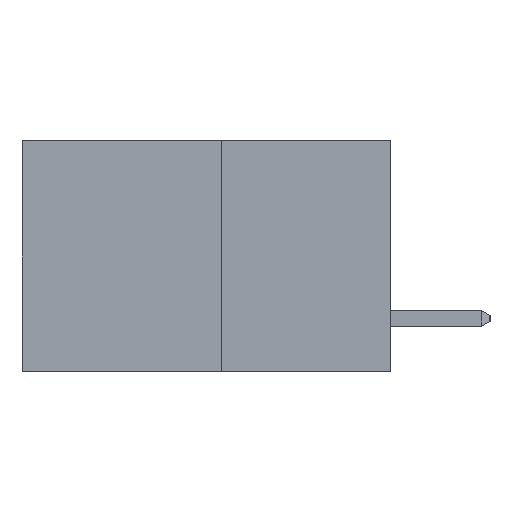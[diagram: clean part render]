
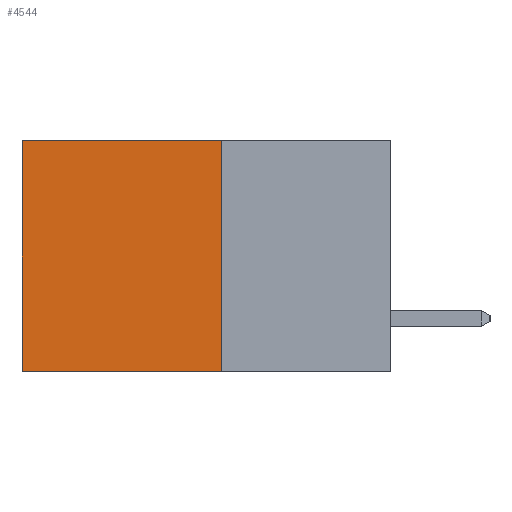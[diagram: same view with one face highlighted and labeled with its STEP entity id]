
A CAD part, left-side view. The second image highlights one B-rep face of the part: STEP entity #4544.
In plain terms, the highlighted planar face has unit normal (-1, 0, 0).
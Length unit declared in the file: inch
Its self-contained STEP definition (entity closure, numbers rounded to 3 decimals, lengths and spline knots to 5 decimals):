
#632 = ORIENTED_EDGE ( 'NONE', *, *, #2432, .T. ) ;
#1020 = VERTEX_POINT ( 'NONE', #12613 ) ;
#1142 = LINE ( 'NONE', #11626, #12280 ) ;
#2432 = EDGE_CURVE ( 'NONE', #9620, #4138, #7521, .T. ) ;
#3687 = VECTOR ( 'NONE', #4342, 39.37008 ) ;
#4007 = ORIENTED_EDGE ( 'NONE', *, *, #14907, .F. ) ;
#4138 = VERTEX_POINT ( 'NONE', #17553 ) ;
#4262 = DIRECTION ( 'NONE',  ( 1., 0., 0. ) ) ;
#4342 = DIRECTION ( 'NONE',  ( 0., 0., -1. ) ) ;
#4544 = ADVANCED_FACE ( 'NONE', ( #16611 ), #11403, .F. ) ;
#4666 = CARTESIAN_POINT ( 'NONE',  ( 0.277, 0.27, 0. ) ) ;
#5407 = EDGE_LOOP ( 'NONE', ( #8310, #11343, #4007, #632 ) ) ;
#7521 = LINE ( 'NONE', #11103, #14602 ) ;
#7532 = LINE ( 'NONE', #10009, #3687 ) ;
#7686 = LINE ( 'NONE', #16466, #8535 ) ;
#7999 = DIRECTION ( 'NONE',  ( 0., 0., -1. ) ) ;
#8310 = ORIENTED_EDGE ( 'NONE', *, *, #10918, .T. ) ;
#8503 = CARTESIAN_POINT ( 'NONE',  ( 0.277, 0.27, -0.37 ) ) ;
#8535 = VECTOR ( 'NONE', #7999, 39.37008 ) ;
#9078 = VERTEX_POINT ( 'NONE', #14856 ) ;
#9620 = VERTEX_POINT ( 'NONE', #4666 ) ;
#10009 = CARTESIAN_POINT ( 'NONE',  ( 0.277, 0.27, -0.37 ) ) ;
#10918 = EDGE_CURVE ( 'NONE', #4138, #9078, #7686, .T. ) ;
#11103 = CARTESIAN_POINT ( 'NONE',  ( 0.277, 0.27, 0. ) ) ;
#11343 = ORIENTED_EDGE ( 'NONE', *, *, #13073, .F. ) ;
#11403 = PLANE ( 'NONE',  #17893 ) ;
#11626 = CARTESIAN_POINT ( 'NONE',  ( 0.277, 0.27, -0.37 ) ) ;
#12280 = VECTOR ( 'NONE', #15766, 39.37008 ) ;
#12613 = CARTESIAN_POINT ( 'NONE',  ( 0.277, 0.27, -0.37 ) ) ;
#13073 = EDGE_CURVE ( 'NONE', #1020, #9078, #1142, .T. ) ;
#13364 = DIRECTION ( 'NONE',  ( 0., 1., 0. ) ) ;
#14242 = DIRECTION ( 'NONE',  ( 0., 0., -1. ) ) ;
#14602 = VECTOR ( 'NONE', #13364, 39.37008 ) ;
#14856 = CARTESIAN_POINT ( 'NONE',  ( 0.277, 0.59, -0.37 ) ) ;
#14907 = EDGE_CURVE ( 'NONE', #9620, #1020, #7532, .T. ) ;
#15766 = DIRECTION ( 'NONE',  ( 0., 1., 0. ) ) ;
#16466 = CARTESIAN_POINT ( 'NONE',  ( 0.277, 0.59, -0.37 ) ) ;
#16611 = FACE_OUTER_BOUND ( 'NONE', #5407, .T. ) ;
#17553 = CARTESIAN_POINT ( 'NONE',  ( 0.277, 0.59, 0. ) ) ;
#17893 = AXIS2_PLACEMENT_3D ( 'NONE', #8503, #4262, #14242 ) ;
